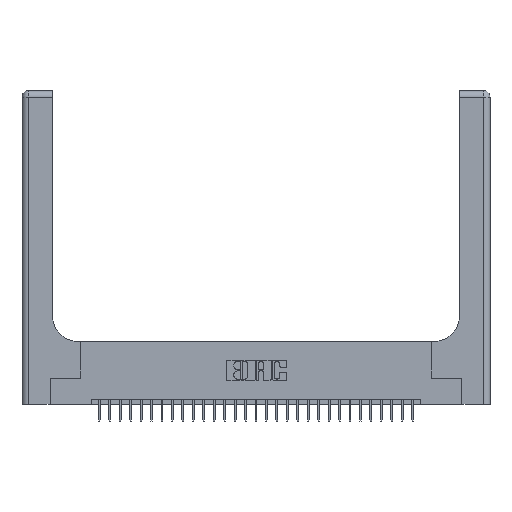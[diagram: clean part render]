
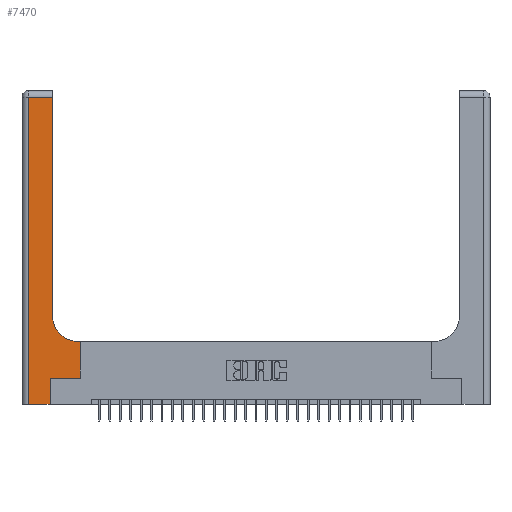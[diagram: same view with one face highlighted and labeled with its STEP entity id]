
A CAD part, top view. The second image highlights one B-rep face of the part: STEP entity #7470.
In plain terms, the highlighted planar face has unit normal (0, 0, 1).
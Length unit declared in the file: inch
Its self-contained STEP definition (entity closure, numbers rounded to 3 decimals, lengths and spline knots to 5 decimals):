
#817 = EDGE_CURVE ( 'NONE', #6560, #7625, #24622, .T. ) ;
#1042 = CARTESIAN_POINT ( 'NONE',  ( 0.06, 2.94, 0.37 ) ) ;
#1047 = CARTESIAN_POINT ( 'NONE',  ( 0., 2.94, 0.37 ) ) ;
#1452 = CARTESIAN_POINT ( 'NONE',  ( 0.5585, 0.6, 0.37 ) ) ;
#1979 = EDGE_CURVE ( 'NONE', #18161, #11750, #16317, .T. ) ;
#3061 = ORIENTED_EDGE ( 'NONE', *, *, #1979, .T. ) ;
#3067 = CARTESIAN_POINT ( 'NONE',  ( 0.5585, 0.25, 0.37 ) ) ;
#3275 = VECTOR ( 'NONE', #6729, 39.37008 ) ;
#3362 = CARTESIAN_POINT ( 'NONE',  ( 0.269, 0., 0.37 ) ) ;
#3804 = CARTESIAN_POINT ( 'NONE',  ( 0.5415, 0.6, 0.37 ) ) ;
#3858 = VECTOR ( 'NONE', #28783, 39.37008 ) ;
#4864 = CARTESIAN_POINT ( 'NONE',  ( 0.2915, 2.94, 0.37 ) ) ;
#4922 = VERTEX_POINT ( 'NONE', #3804 ) ;
#5296 = ORIENTED_EDGE ( 'NONE', *, *, #817, .T. ) ;
#5399 = EDGE_CURVE ( 'NONE', #7625, #18161, #23548, .T. ) ;
#5430 = VECTOR ( 'NONE', #14296, 39.37008 ) ;
#5522 = CARTESIAN_POINT ( 'NONE',  ( 0.06, 0., 0.37 ) ) ;
#5620 = LINE ( 'NONE', #30095, #29646 ) ;
#5644 = EDGE_CURVE ( 'NONE', #11373, #4922, #15587, .T. ) ;
#6418 = DIRECTION ( 'NONE',  ( -1., 0., 0. ) ) ;
#6560 = VERTEX_POINT ( 'NONE', #5522 ) ;
#6729 = DIRECTION ( 'NONE',  ( 0., 1., 0. ) ) ;
#6770 = DIRECTION ( 'NONE',  ( 1., 0., 0. ) ) ;
#6840 = DIRECTION ( 'NONE',  ( 0., 0., -1. ) ) ;
#7148 = VERTEX_POINT ( 'NONE', #23266 ) ;
#7261 = DIRECTION ( 'NONE',  ( 0., -1., 0. ) ) ;
#7470 = ADVANCED_FACE ( 'NONE', ( #14352 ), #23151, .F. ) ;
#7625 = VERTEX_POINT ( 'NONE', #3362 ) ;
#7706 = EDGE_CURVE ( 'NONE', #7148, #11614, #15479, .T. ) ;
#8957 = EDGE_CURVE ( 'NONE', #11750, #11373, #27786, .T. ) ;
#9171 = CARTESIAN_POINT ( 'NONE',  ( 0.5585, 0.25, 0.37 ) ) ;
#9231 = VECTOR ( 'NONE', #6418, 39.37008 ) ;
#9329 = ORIENTED_EDGE ( 'NONE', *, *, #10834, .T. ) ;
#10834 = EDGE_CURVE ( 'NONE', #13092, #6560, #5620, .T. ) ;
#10836 = ORIENTED_EDGE ( 'NONE', *, *, #7706, .T. ) ;
#11373 = VERTEX_POINT ( 'NONE', #1452 ) ;
#11614 = VERTEX_POINT ( 'NONE', #4864 ) ;
#11750 = VERTEX_POINT ( 'NONE', #3067 ) ;
#12332 = ORIENTED_EDGE ( 'NONE', *, *, #8957, .T. ) ;
#13092 = VERTEX_POINT ( 'NONE', #1042 ) ;
#13826 = CARTESIAN_POINT ( 'NONE',  ( 0.5415, 0.85, 0.37 ) ) ;
#14296 = DIRECTION ( 'NONE',  ( 1., 0., 0. ) ) ;
#14352 = FACE_OUTER_BOUND ( 'NONE', #30760, .T. ) ;
#14946 = ORIENTED_EDGE ( 'NONE', *, *, #5399, .T. ) ;
#15479 = LINE ( 'NONE', #16701, #3858 ) ;
#15526 = EDGE_CURVE ( 'NONE', #11614, #13092, #24193, .T. ) ;
#15587 = LINE ( 'NONE', #20849, #9231 ) ;
#16317 = LINE ( 'NONE', #16497, #5430 ) ;
#16487 = DIRECTION ( 'NONE',  ( -1., 0., 0. ) ) ;
#16497 = CARTESIAN_POINT ( 'NONE',  ( 0.269, 0.25, 0.37 ) ) ;
#16594 = AXIS2_PLACEMENT_3D ( 'NONE', #21291, #6840, #16487 ) ;
#16701 = CARTESIAN_POINT ( 'NONE',  ( 0.2915, 3., 0.37 ) ) ;
#16733 = CARTESIAN_POINT ( 'NONE',  ( 0.269, 0.25, 0.37 ) ) ;
#17422 = ORIENTED_EDGE ( 'NONE', *, *, #15526, .T. ) ;
#17765 = VECTOR ( 'NONE', #20247, 39.37008 ) ;
#18161 = VERTEX_POINT ( 'NONE', #16733 ) ;
#20247 = DIRECTION ( 'NONE',  ( -1., 0., 0. ) ) ;
#20849 = CARTESIAN_POINT ( 'NONE',  ( 0.2915, 0.6, 0.37 ) ) ;
#21291 = CARTESIAN_POINT ( 'NONE',  ( 0., 3., 0.37 ) ) ;
#21437 = CIRCLE ( 'NONE', #29191, 0.25 ) ;
#21450 = VECTOR ( 'NONE', #21495, 39.37008 ) ;
#21495 = DIRECTION ( 'NONE',  ( 0., 1., 0. ) ) ;
#23151 = PLANE ( 'NONE',  #16594 ) ;
#23266 = CARTESIAN_POINT ( 'NONE',  ( 0.2915, 0.85, 0.37 ) ) ;
#23548 = LINE ( 'NONE', #23788, #3275 ) ;
#23788 = CARTESIAN_POINT ( 'NONE',  ( 0.269, 0., 0.37 ) ) ;
#24193 = LINE ( 'NONE', #1047, #17765 ) ;
#24622 = LINE ( 'NONE', #29082, #27619 ) ;
#26245 = ORIENTED_EDGE ( 'NONE', *, *, #29822, .T. ) ;
#26784 = ORIENTED_EDGE ( 'NONE', *, *, #5644, .T. ) ;
#27619 = VECTOR ( 'NONE', #28981, 39.37008 ) ;
#27786 = LINE ( 'NONE', #9171, #21450 ) ;
#28330 = DIRECTION ( 'NONE',  ( 0., 0., -1. ) ) ;
#28783 = DIRECTION ( 'NONE',  ( 0., 1., 0. ) ) ;
#28981 = DIRECTION ( 'NONE',  ( 1., 0., 0. ) ) ;
#29082 = CARTESIAN_POINT ( 'NONE',  ( 0., 0., 0.37 ) ) ;
#29191 = AXIS2_PLACEMENT_3D ( 'NONE', #13826, #28330, #6770 ) ;
#29646 = VECTOR ( 'NONE', #7261, 39.37008 ) ;
#29822 = EDGE_CURVE ( 'NONE', #4922, #7148, #21437, .T. ) ;
#30095 = CARTESIAN_POINT ( 'NONE',  ( 0.06, 3., 0.37 ) ) ;
#30760 = EDGE_LOOP ( 'NONE', ( #10836, #17422, #9329, #5296, #14946, #3061, #12332, #26784, #26245 ) ) ;
